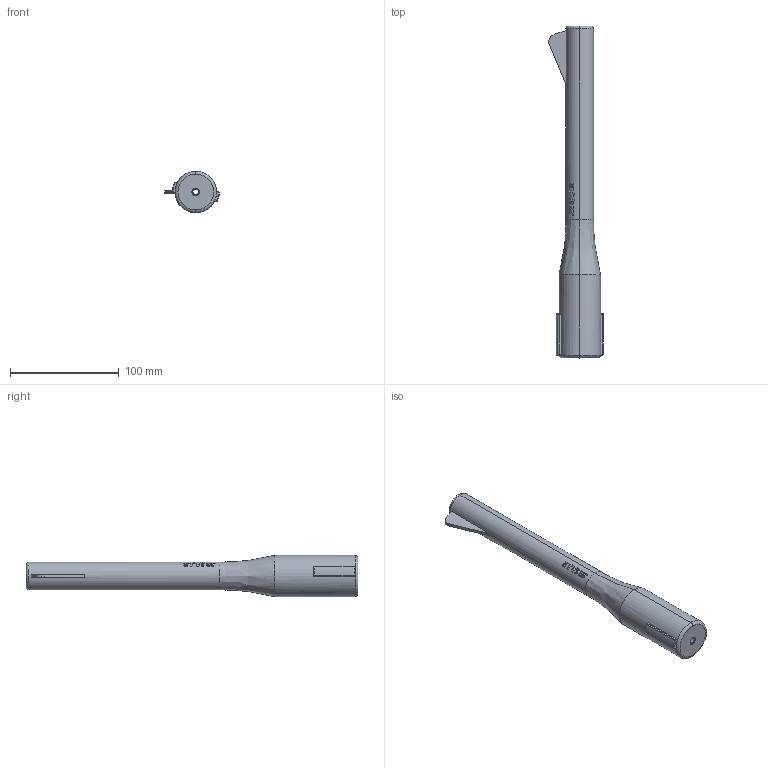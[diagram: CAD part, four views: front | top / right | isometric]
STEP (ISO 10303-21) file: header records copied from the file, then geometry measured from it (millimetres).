
FILE_DESCRIPTION (( 'STEP AP214' ), '1' );
FILE_NAME ('barrel12.STEP', '2013-10-27T06:43:17', ( 'Matt' ), ( '' ), 'SwSTEP 2.0', 'SolidWorks 2013', '' );
FILE_SCHEMA (( 'AUTOMOTIVE_DESIGN' ));
Length unit declared in the file: inch
Products named in the file (1): barrel12
Bounding box: 50.13 x 304.8 x 38.1 mm (x, y, z)
Volume: 204756.3 mm3; surface area: 37878.6 mm2
Topology: 1 solids, 1 shells, 183 faces, 479 edges, 302 vertices
Faces by surface type: bspline 69, plane 52, cylinder 44, torus 8, sphere 8, cone 2
Entity records: 17439 total; most frequent: CARTESIAN_POINT 13639, ORIENTED_EDGE 942, DIRECTION 559, EDGE_CURVE 471, VERTEX_POINT 302, AXIS2_PLACEMENT_3D 221, EDGE_LOOP 197, ADVANCED_FACE 183
